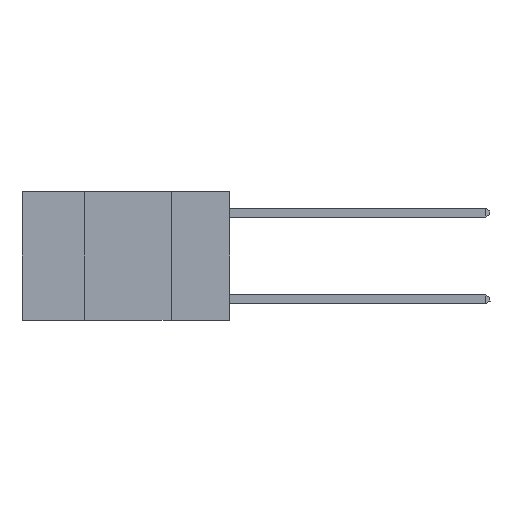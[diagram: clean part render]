
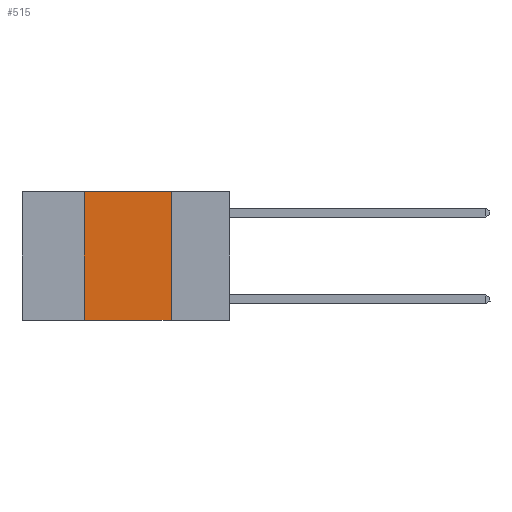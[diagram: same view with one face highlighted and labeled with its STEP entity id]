
A CAD part, left-side view. The second image highlights one B-rep face of the part: STEP entity #515.
In plain terms, the highlighted planar face has unit normal (-1, 0, 0).
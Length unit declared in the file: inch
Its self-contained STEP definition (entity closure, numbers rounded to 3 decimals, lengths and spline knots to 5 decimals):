
#515 = ADVANCED_FACE ( 'NONE', ( #27908 ), #14875, .F. ) ;
#1004 = DIRECTION ( 'NONE',  ( 0., -1., 0. ) ) ;
#1759 = EDGE_CURVE ( 'NONE', #13145, #15521, #26737, .T. ) ;
#3349 = EDGE_CURVE ( 'NONE', #23959, #21515, #4807, .T. ) ;
#3582 = CARTESIAN_POINT ( 'NONE',  ( 0., 0.17, 0. ) ) ;
#4245 = CARTESIAN_POINT ( 'NONE',  ( 0., 0.42, 0. ) ) ;
#4807 = LINE ( 'NONE', #3582, #17926 ) ;
#5192 = DIRECTION ( 'NONE',  ( 0., -1., 0. ) ) ;
#5224 = CARTESIAN_POINT ( 'NONE',  ( 0., 0.42, 0. ) ) ;
#6807 = LINE ( 'NONE', #12940, #18834 ) ;
#7423 = DIRECTION ( 'NONE',  ( 0., 0., 1. ) ) ;
#11105 = CARTESIAN_POINT ( 'NONE',  ( 0., 0.17, 0. ) ) ;
#12935 = ORIENTED_EDGE ( 'NONE', *, *, #27976, .F. ) ;
#12940 = CARTESIAN_POINT ( 'NONE',  ( 0., 0.6, 0. ) ) ;
#13145 = VERTEX_POINT ( 'NONE', #28121 ) ;
#14161 = AXIS2_PLACEMENT_3D ( 'NONE', #14869, #14733, #14629 ) ;
#14629 = DIRECTION ( 'NONE',  ( 0., 0., -1. ) ) ;
#14733 = DIRECTION ( 'NONE',  ( 1., 0., 0. ) ) ;
#14869 = CARTESIAN_POINT ( 'NONE',  ( 0., 0.6, 0. ) ) ;
#14875 = PLANE ( 'NONE',  #14161 ) ;
#15521 = VERTEX_POINT ( 'NONE', #4245 ) ;
#17786 = ORIENTED_EDGE ( 'NONE', *, *, #3349, .F. ) ;
#17926 = VECTOR ( 'NONE', #17945, 39.37008 ) ;
#17945 = DIRECTION ( 'NONE',  ( 0., 0., -1. ) ) ;
#18182 = LINE ( 'NONE', #21959, #23029 ) ;
#18834 = VECTOR ( 'NONE', #1004, 39.37008 ) ;
#20263 = EDGE_LOOP ( 'NONE', ( #17786, #12935, #26691, #29296 ) ) ;
#20995 = CARTESIAN_POINT ( 'NONE',  ( 0., 0.17, -0.37 ) ) ;
#21515 = VERTEX_POINT ( 'NONE', #20995 ) ;
#21959 = CARTESIAN_POINT ( 'NONE',  ( 0., 0.6, -0.37 ) ) ;
#23029 = VECTOR ( 'NONE', #5192, 39.37008 ) ;
#23959 = VERTEX_POINT ( 'NONE', #11105 ) ;
#26022 = VECTOR ( 'NONE', #7423, 39.37008 ) ;
#26292 = EDGE_CURVE ( 'NONE', #13145, #21515, #18182, .T. ) ;
#26691 = ORIENTED_EDGE ( 'NONE', *, *, #1759, .F. ) ;
#26737 = LINE ( 'NONE', #5224, #26022 ) ;
#27908 = FACE_OUTER_BOUND ( 'NONE', #20263, .T. ) ;
#27976 = EDGE_CURVE ( 'NONE', #15521, #23959, #6807, .T. ) ;
#28121 = CARTESIAN_POINT ( 'NONE',  ( 0., 0.42, -0.37 ) ) ;
#29296 = ORIENTED_EDGE ( 'NONE', *, *, #26292, .T. ) ;
